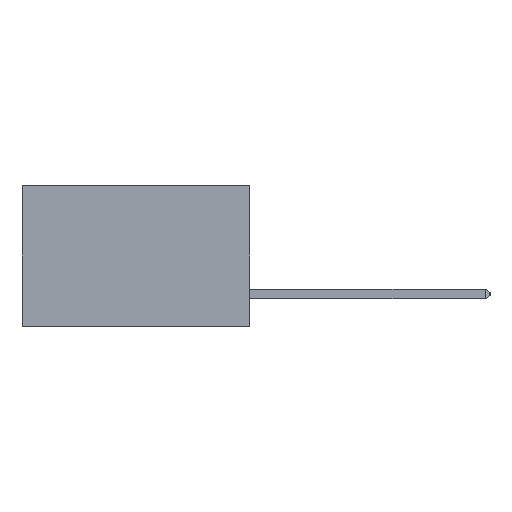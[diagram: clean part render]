
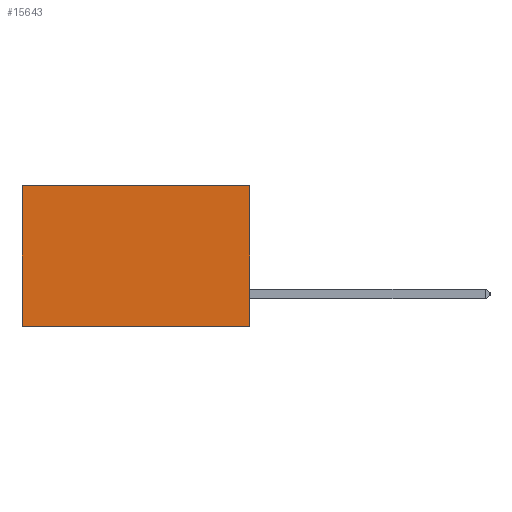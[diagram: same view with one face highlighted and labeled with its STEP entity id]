
A CAD part, left-side view. The second image highlights one B-rep face of the part: STEP entity #15643.
In plain terms, the highlighted planar face has unit normal (-1, 0, 0).
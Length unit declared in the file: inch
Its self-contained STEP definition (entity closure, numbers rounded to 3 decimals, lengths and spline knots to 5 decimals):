
#512 = FACE_OUTER_BOUND ( 'NONE', #16177, .T. ) ;
#3818 = CARTESIAN_POINT ( 'NONE',  ( 0.2875, 0.6, -0.37 ) ) ;
#4254 = PLANE ( 'NONE',  #24717 ) ;
#4945 = VERTEX_POINT ( 'NONE', #18198 ) ;
#5854 = VECTOR ( 'NONE', #9329, 39.37008 ) ;
#6953 = CARTESIAN_POINT ( 'NONE',  ( 0.2875, 0., -0.37 ) ) ;
#7306 = LINE ( 'NONE', #6953, #5854 ) ;
#8952 = DIRECTION ( 'NONE',  ( 0., 0., -1. ) ) ;
#9218 = CARTESIAN_POINT ( 'NONE',  ( 0.2875, 0., 0. ) ) ;
#9329 = DIRECTION ( 'NONE',  ( 0., 1., 0. ) ) ;
#10144 = CARTESIAN_POINT ( 'NONE',  ( 0.2875, 0.6, 0. ) ) ;
#11244 = ORIENTED_EDGE ( 'NONE', *, *, #12112, .T. ) ;
#11673 = ORIENTED_EDGE ( 'NONE', *, *, #19767, .T. ) ;
#11868 = DIRECTION ( 'NONE',  ( 0., 0., -1. ) ) ;
#12112 = EDGE_CURVE ( 'NONE', #23572, #14972, #29756, .T. ) ;
#13296 = EDGE_CURVE ( 'NONE', #4945, #23148, #21032, .T. ) ;
#14217 = VECTOR ( 'NONE', #27772, 39.37008 ) ;
#14972 = VERTEX_POINT ( 'NONE', #3818 ) ;
#15643 = ADVANCED_FACE ( 'NONE', ( #512 ), #4254, .F. ) ;
#16177 = EDGE_LOOP ( 'NONE', ( #11244, #17584, #29961, #11673 ) ) ;
#17584 = ORIENTED_EDGE ( 'NONE', *, *, #21579, .F. ) ;
#17868 = DIRECTION ( 'NONE',  ( 0., 1., 0. ) ) ;
#18198 = CARTESIAN_POINT ( 'NONE',  ( 0.2875, 0., 0. ) ) ;
#18696 = CARTESIAN_POINT ( 'NONE',  ( 0.2875, 0.6, 0. ) ) ;
#19767 = EDGE_CURVE ( 'NONE', #4945, #23572, #26992, .T. ) ;
#20097 = VECTOR ( 'NONE', #17868, 39.37008 ) ;
#20183 = CARTESIAN_POINT ( 'NONE',  ( 0.2875, 0., -0.37 ) ) ;
#20488 = CARTESIAN_POINT ( 'NONE',  ( 0.2875, 0., 0. ) ) ;
#21032 = LINE ( 'NONE', #9218, #14217 ) ;
#21579 = EDGE_CURVE ( 'NONE', #23148, #14972, #7306, .T. ) ;
#22531 = CARTESIAN_POINT ( 'NONE',  ( 0.2875, 0., 0. ) ) ;
#22838 = DIRECTION ( 'NONE',  ( 1., 0., 0. ) ) ;
#23148 = VERTEX_POINT ( 'NONE', #20183 ) ;
#23572 = VERTEX_POINT ( 'NONE', #10144 ) ;
#23657 = VECTOR ( 'NONE', #11868, 39.37008 ) ;
#24717 = AXIS2_PLACEMENT_3D ( 'NONE', #20488, #22838, #8952 ) ;
#26992 = LINE ( 'NONE', #22531, #20097 ) ;
#27772 = DIRECTION ( 'NONE',  ( 0., 0., -1. ) ) ;
#29756 = LINE ( 'NONE', #18696, #23657 ) ;
#29961 = ORIENTED_EDGE ( 'NONE', *, *, #13296, .F. ) ;
